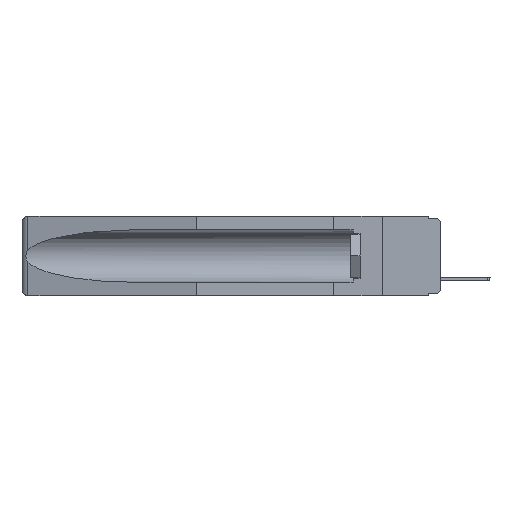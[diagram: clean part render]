
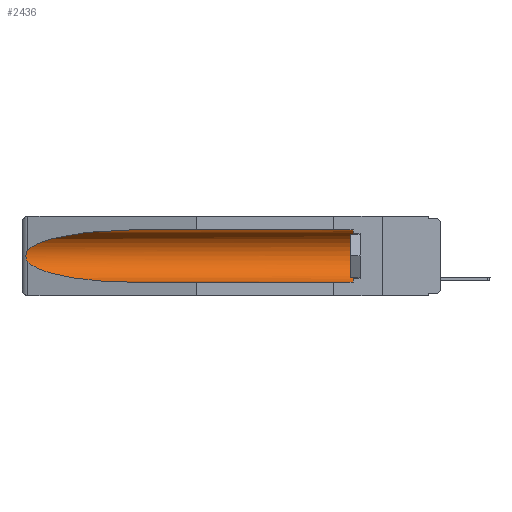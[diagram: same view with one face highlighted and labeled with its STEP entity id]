
A CAD part, left-side view. The second image highlights one B-rep face of the part: STEP entity #2436.
In plain terms, the highlighted cylindrical face has radius 2.857 mm (diameter 5.715 mm), a partial arc.
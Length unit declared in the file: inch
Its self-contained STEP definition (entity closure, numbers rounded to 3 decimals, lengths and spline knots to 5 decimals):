
#172 = CARTESIAN_POINT ( 'NONE',  ( 0.155, 0.126, -0.1715 ) ) ;
#746 = LINE ( 'NONE', #1264, #9026 ) ;
#1264 = CARTESIAN_POINT ( 'NONE',  ( 0.155, -0.30754, -0.284 ) ) ;
#1507 = EDGE_CURVE ( 'NONE', #6086, #8325, #12927, .T. ) ;
#2111 = B_SPLINE_CURVE_WITH_KNOTS ( 'NONE', 3,
 ( #19054, #11587, #2327, #5180, #11389, #6691, #19120, #16014, #2254, #17504 ),
 .UNSPECIFIED., .F., .F.,
 ( 4, 2, 2, 2, 4 ),
 ( 0., 0.00029, 0.00058, 0.00087, 0.00117 ),
 .UNSPECIFIED. ) ;
#2117 = DIRECTION ( 'NONE',  ( 0., 0., 1. ) ) ;
#2254 = CARTESIAN_POINT ( 'NONE',  ( 0.26597, 1.5296, -0.19026 ) ) ;
#2312 = EDGE_CURVE ( 'NONE', #7281, #3149, #17394, .T. ) ;
#2327 = CARTESIAN_POINT ( 'NONE',  ( 0.26654, 1.53092, -0.15636 ) ) ;
#2400 = EDGE_CURVE ( 'NONE', #3149, #6086, #2111, .T. ) ;
#2436 = ADVANCED_FACE ( 'NONE', ( #5905 ), #3945, .F. ) ;
#2547 = CARTESIAN_POINT ( 'NONE',  ( 0.155, 1.07973, -0.284 ) ) ;
#3133 = CARTESIAN_POINT ( 'NONE',  ( 0.26537, 1.52718, -0.14972 ) ) ;
#3149 = VERTEX_POINT ( 'NONE', #3133 ) ;
#3696 = CARTESIAN_POINT ( 'NONE',  ( 0.155, -0.30754, -0.1715 ) ) ;
#3900 = EDGE_CURVE ( 'NONE', #9919, #7281, #5867, .T. ) ;
#3945 = CYLINDRICAL_SURFACE ( 'NONE', #8820, 0.1125 ) ;
#4913 = CARTESIAN_POINT ( 'NONE',  ( 0.21114, 1.30732, -0.059 ) ) ;
#5180 = CARTESIAN_POINT ( 'NONE',  ( 0.2673, 1.5327, -0.16383 ) ) ;
#5766 = DIRECTION ( 'NONE',  ( 0., 1., 0. ) ) ;
#5867 = LINE ( 'NONE', #17573, #13619 ) ;
#5905 = FACE_OUTER_BOUND ( 'NONE', #11233, .T. ) ;
#5947 = CARTESIAN_POINT ( 'NONE',  ( 0.21114, 1.30732, -0.284 ) ) ;
#6086 = VERTEX_POINT ( 'NONE', #10833 ) ;
#6691 = CARTESIAN_POINT ( 'NONE',  ( 0.2675, 1.53308, -0.17534 ) ) ;
#7074 = CARTESIAN_POINT ( 'NONE',  ( 0.155, 0.126, -0.059 ) ) ;
#7281 = VERTEX_POINT ( 'NONE', #18951 ) ;
#7676 = EDGE_CURVE ( 'NONE', #19526, #8325, #746, .T. ) ;
#7858 = DIRECTION ( 'NONE',  ( 0., 0., 1. ) ) ;
#8258 = DIRECTION ( 'NONE',  ( 0., 1., 0. ) ) ;
#8325 = VERTEX_POINT ( 'NONE', #13722 ) ;
#8820 = AXIS2_PLACEMENT_3D ( 'NONE', #3696, #8258, #2117 ) ;
#9026 = VECTOR ( 'NONE', #5766, 39.37008 ) ;
#9052 = ORIENTED_EDGE ( 'NONE', *, *, #3900, .T. ) ;
#9102 = CARTESIAN_POINT ( 'NONE',  ( 0.155, 0.126, -0.284 ) ) ;
#9683 = CARTESIAN_POINT ( 'NONE',  ( 0.155, 1.07973, -0.059 ) ) ;
#9919 = VERTEX_POINT ( 'NONE', #7074 ) ;
#10675 = ORIENTED_EDGE ( 'NONE', *, *, #7676, .F. ) ;
#10833 = CARTESIAN_POINT ( 'NONE',  ( 0.26537, 1.52718, -0.19328 ) ) ;
#10874 = DIRECTION ( 'NONE',  ( 0., -1., 0. ) ) ;
#11233 = EDGE_LOOP ( 'NONE', ( #12559, #17727, #15958, #10675, #18470, #9052 ) ) ;
#11389 = CARTESIAN_POINT ( 'NONE',  ( 0.2675, 1.53308, -0.16763 ) ) ;
#11524 = DIRECTION ( 'NONE',  ( 0., 1., 0. ) ) ;
#11587 = CARTESIAN_POINT ( 'NONE',  ( 0.26597, 1.52961, -0.15275 ) ) ;
#11912 = AXIS2_PLACEMENT_3D ( 'NONE', #172, #10874, #7858 ) ;
#12559 = ORIENTED_EDGE ( 'NONE', *, *, #2312, .T. ) ;
#12614 = EDGE_CURVE ( 'NONE', #19526, #9919, #15185, .T. ) ;
#12732 = CARTESIAN_POINT ( 'NONE',  ( 0.26537, 1.52718, -0.14972 ) ) ;
#12927 =( BOUNDED_CURVE ( )  B_SPLINE_CURVE ( 3, ( #15077, #15207, #5947, #2547 ),
 .UNSPECIFIED., .F., .F. ) 
 B_SPLINE_CURVE_WITH_KNOTS ( ( 4, 4 ),
 ( 0.1948, 1.5708 ),
 .UNSPECIFIED. ) 
 CURVE ( )  GEOMETRIC_REPRESENTATION_ITEM ( )  RATIONAL_B_SPLINE_CURVE ( ( 1., 0.848, 0.848, 1. ) ) 
 REPRESENTATION_ITEM ( '' )  );
#13619 = VECTOR ( 'NONE', #11524, 39.37008 ) ;
#13722 = CARTESIAN_POINT ( 'NONE',  ( 0.155, 1.07973, -0.284 ) ) ;
#15077 = CARTESIAN_POINT ( 'NONE',  ( 0.26537, 1.52718, -0.19328 ) ) ;
#15185 = CIRCLE ( 'NONE', #11912, 0.1125 ) ;
#15207 = CARTESIAN_POINT ( 'NONE',  ( 0.25451, 1.48313, -0.24835 ) ) ;
#15958 = ORIENTED_EDGE ( 'NONE', *, *, #1507, .T. ) ;
#16014 = CARTESIAN_POINT ( 'NONE',  ( 0.26655, 1.53094, -0.18657 ) ) ;
#17394 =( BOUNDED_CURVE ( )  B_SPLINE_CURVE ( 3, ( #9683, #4913, #18787, #12732 ),
 .UNSPECIFIED., .F., .F. ) 
 B_SPLINE_CURVE_WITH_KNOTS ( ( 4, 4 ),
 ( 4.71239, 6.08839 ),
 .UNSPECIFIED. ) 
 CURVE ( )  GEOMETRIC_REPRESENTATION_ITEM ( )  RATIONAL_B_SPLINE_CURVE ( ( 1., 0.848, 0.848, 1. ) ) 
 REPRESENTATION_ITEM ( '' )  );
#17504 = CARTESIAN_POINT ( 'NONE',  ( 0.26537, 1.52718, -0.19328 ) ) ;
#17573 = CARTESIAN_POINT ( 'NONE',  ( 0.155, -0.30754, -0.059 ) ) ;
#17727 = ORIENTED_EDGE ( 'NONE', *, *, #2400, .T. ) ;
#18470 = ORIENTED_EDGE ( 'NONE', *, *, #12614, .T. ) ;
#18787 = CARTESIAN_POINT ( 'NONE',  ( 0.25451, 1.48313, -0.09465 ) ) ;
#18951 = CARTESIAN_POINT ( 'NONE',  ( 0.155, 1.07973, -0.059 ) ) ;
#19054 = CARTESIAN_POINT ( 'NONE',  ( 0.26537, 1.52718, -0.14972 ) ) ;
#19120 = CARTESIAN_POINT ( 'NONE',  ( 0.2673, 1.53269, -0.17917 ) ) ;
#19526 = VERTEX_POINT ( 'NONE', #9102 ) ;
